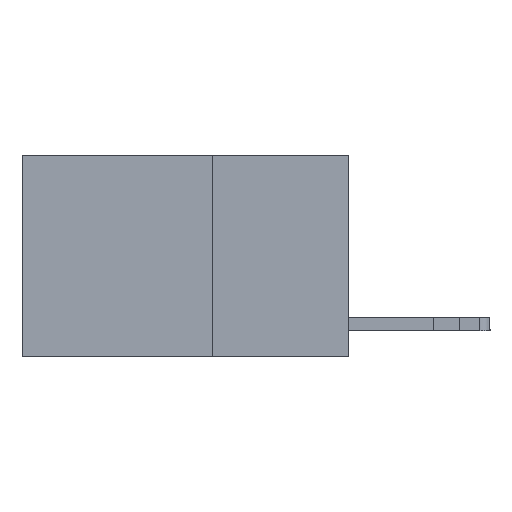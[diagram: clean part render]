
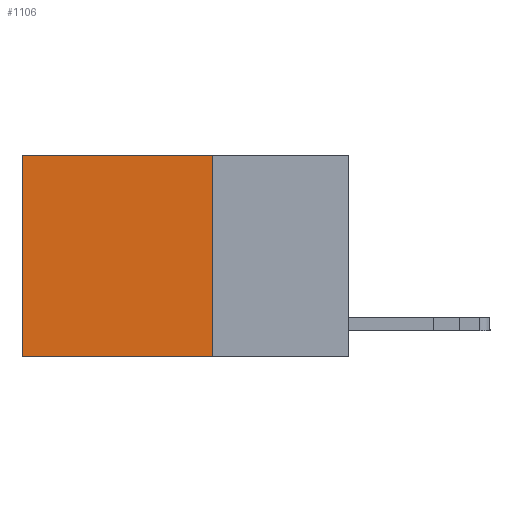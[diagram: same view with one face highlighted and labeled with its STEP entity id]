
A CAD part, left-side view. The second image highlights one B-rep face of the part: STEP entity #1106.
In plain terms, the highlighted planar face has unit normal (-1, 0, 0).
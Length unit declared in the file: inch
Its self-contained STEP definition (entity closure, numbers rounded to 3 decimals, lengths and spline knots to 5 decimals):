
#54 = LINE ( 'NONE', #9757, #13764 ) ;
#126 = PLANE ( 'NONE',  #12013 ) ;
#182 = LINE ( 'NONE', #4994, #14667 ) ;
#764 = ORIENTED_EDGE ( 'NONE', *, *, #12676, .F. ) ;
#1106 = ADVANCED_FACE ( 'NONE', ( #12111 ), #126, .F. ) ;
#1340 = VERTEX_POINT ( 'NONE', #5565 ) ;
#3327 = EDGE_CURVE ( 'NONE', #4378, #1340, #8217, .T. ) ;
#3825 = DIRECTION ( 'NONE',  ( 0., 1., 0. ) ) ;
#4378 = VERTEX_POINT ( 'NONE', #14906 ) ;
#4858 = DIRECTION ( 'NONE',  ( 1., 0., 0. ) ) ;
#4994 = CARTESIAN_POINT ( 'NONE',  ( 0.2625, 0.6, 0. ) ) ;
#5381 = CARTESIAN_POINT ( 'NONE',  ( 0.2625, 0.25, -0.37 ) ) ;
#5565 = CARTESIAN_POINT ( 'NONE',  ( 0.2625, 0.25, -0.37 ) ) ;
#6152 = ORIENTED_EDGE ( 'NONE', *, *, #9522, .T. ) ;
#6254 = DIRECTION ( 'NONE',  ( 0., 0., -1. ) ) ;
#7045 = CARTESIAN_POINT ( 'NONE',  ( 0.2625, 0.25, 0. ) ) ;
#7200 = VECTOR ( 'NONE', #10184, 39.37008 ) ;
#7237 = DIRECTION ( 'NONE',  ( 0., 0., -1. ) ) ;
#8217 = LINE ( 'NONE', #7045, #14617 ) ;
#8701 = ORIENTED_EDGE ( 'NONE', *, *, #14875, .T. ) ;
#9510 = CARTESIAN_POINT ( 'NONE',  ( 0.2625, 0.6, -0.37 ) ) ;
#9522 = EDGE_CURVE ( 'NONE', #10926, #13511, #182, .T. ) ;
#9757 = CARTESIAN_POINT ( 'NONE',  ( 0.2625, 0.25, 0. ) ) ;
#10184 = DIRECTION ( 'NONE',  ( 0., 1., 0. ) ) ;
#10926 = VERTEX_POINT ( 'NONE', #11225 ) ;
#11225 = CARTESIAN_POINT ( 'NONE',  ( 0.2625, 0.6, 0. ) ) ;
#11839 = DIRECTION ( 'NONE',  ( 0., 0., -1. ) ) ;
#12013 = AXIS2_PLACEMENT_3D ( 'NONE', #14441, #4858, #7237 ) ;
#12111 = FACE_OUTER_BOUND ( 'NONE', #14102, .T. ) ;
#12676 = EDGE_CURVE ( 'NONE', #1340, #13511, #13704, .T. ) ;
#13511 = VERTEX_POINT ( 'NONE', #9510 ) ;
#13704 = LINE ( 'NONE', #5381, #7200 ) ;
#13764 = VECTOR ( 'NONE', #3825, 39.37008 ) ;
#14102 = EDGE_LOOP ( 'NONE', ( #6152, #764, #15098, #8701 ) ) ;
#14441 = CARTESIAN_POINT ( 'NONE',  ( 0.2625, 0.25, 0. ) ) ;
#14617 = VECTOR ( 'NONE', #11839, 39.37008 ) ;
#14667 = VECTOR ( 'NONE', #6254, 39.37008 ) ;
#14875 = EDGE_CURVE ( 'NONE', #4378, #10926, #54, .T. ) ;
#14906 = CARTESIAN_POINT ( 'NONE',  ( 0.2625, 0.25, 0. ) ) ;
#15098 = ORIENTED_EDGE ( 'NONE', *, *, #3327, .F. ) ;
